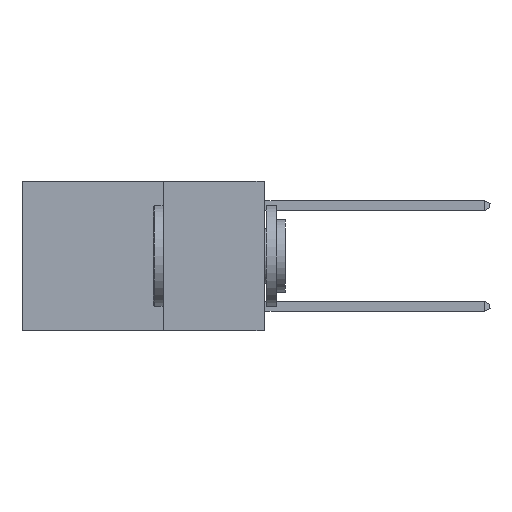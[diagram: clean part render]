
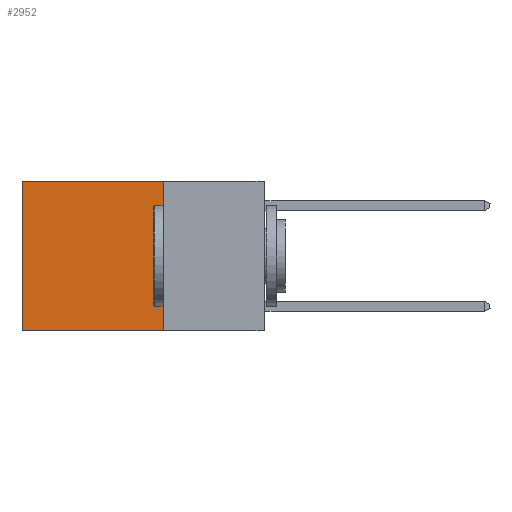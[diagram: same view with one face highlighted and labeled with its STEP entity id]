
A CAD part, left-side view. The second image highlights one B-rep face of the part: STEP entity #2952.
In plain terms, the highlighted planar face has unit normal (-1, 0, 0).
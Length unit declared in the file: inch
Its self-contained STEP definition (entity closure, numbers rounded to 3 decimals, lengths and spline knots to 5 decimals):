
#138 = CARTESIAN_POINT ( 'NONE',  ( 0.2625, 0.25, 0. ) ) ;
#767 = CARTESIAN_POINT ( 'NONE',  ( 0.2625, 0.25, 0. ) ) ;
#833 = AXIS2_PLACEMENT_3D ( 'NONE', #767, #2411, #2355 ) ;
#944 = CARTESIAN_POINT ( 'NONE',  ( 0.2625, 0.6, 0. ) ) ;
#1382 = EDGE_CURVE ( 'NONE', #9737, #2724, #3249, .T. ) ;
#1823 = ORIENTED_EDGE ( 'NONE', *, *, #4301, .F. ) ;
#2355 = DIRECTION ( 'NONE',  ( 0., 0., -1. ) ) ;
#2411 = DIRECTION ( 'NONE',  ( 1., 0., 0. ) ) ;
#2544 = EDGE_CURVE ( 'NONE', #9737, #4849, #4011, .T. ) ;
#2575 = DIRECTION ( 'NONE',  ( 0., 0., -1. ) ) ;
#2724 = VERTEX_POINT ( 'NONE', #2727 ) ;
#2727 = CARTESIAN_POINT ( 'NONE',  ( 0.2625, 0.6, 0. ) ) ;
#2952 = ADVANCED_FACE ( 'NONE', ( #7305 ), #7984, .F. ) ;
#3095 = VECTOR ( 'NONE', #4284, 39.37008 ) ;
#3155 = CARTESIAN_POINT ( 'NONE',  ( 0.2625, 0.6, -0.37 ) ) ;
#3249 = LINE ( 'NONE', #8066, #4348 ) ;
#3943 = DIRECTION ( 'NONE',  ( 0., 1., 0. ) ) ;
#4011 = LINE ( 'NONE', #138, #4884 ) ;
#4284 = DIRECTION ( 'NONE',  ( 0., 0., -1. ) ) ;
#4301 = EDGE_CURVE ( 'NONE', #4849, #4329, #9337, .T. ) ;
#4329 = VERTEX_POINT ( 'NONE', #3155 ) ;
#4348 = VECTOR ( 'NONE', #8639, 39.37008 ) ;
#4849 = VERTEX_POINT ( 'NONE', #8273 ) ;
#4884 = VECTOR ( 'NONE', #2575, 39.37008 ) ;
#4886 = ORIENTED_EDGE ( 'NONE', *, *, #1382, .T. ) ;
#5036 = ORIENTED_EDGE ( 'NONE', *, *, #6822, .T. ) ;
#5068 = LINE ( 'NONE', #944, #3095 ) ;
#6422 = EDGE_LOOP ( 'NONE', ( #5036, #1823, #8676, #4886 ) ) ;
#6822 = EDGE_CURVE ( 'NONE', #2724, #4329, #5068, .T. ) ;
#7305 = FACE_OUTER_BOUND ( 'NONE', #6422, .T. ) ;
#7984 = PLANE ( 'NONE',  #833 ) ;
#8066 = CARTESIAN_POINT ( 'NONE',  ( 0.2625, 0.25, 0. ) ) ;
#8084 = VECTOR ( 'NONE', #3943, 39.37008 ) ;
#8273 = CARTESIAN_POINT ( 'NONE',  ( 0.2625, 0.25, -0.37 ) ) ;
#8639 = DIRECTION ( 'NONE',  ( 0., 1., 0. ) ) ;
#8676 = ORIENTED_EDGE ( 'NONE', *, *, #2544, .F. ) ;
#8766 = CARTESIAN_POINT ( 'NONE',  ( 0.2625, 0.25, -0.37 ) ) ;
#9337 = LINE ( 'NONE', #8766, #8084 ) ;
#9737 = VERTEX_POINT ( 'NONE', #9962 ) ;
#9962 = CARTESIAN_POINT ( 'NONE',  ( 0.2625, 0.25, 0. ) ) ;
